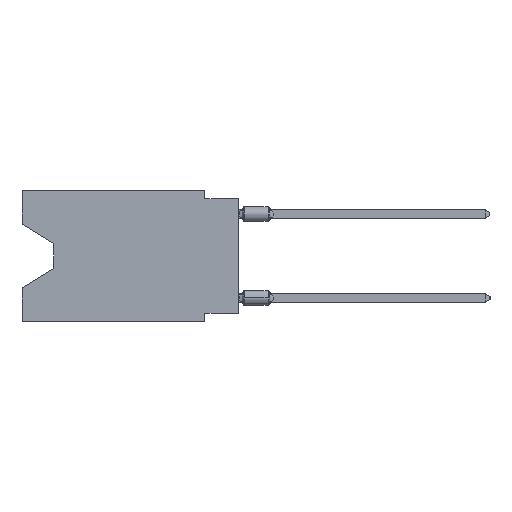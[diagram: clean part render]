
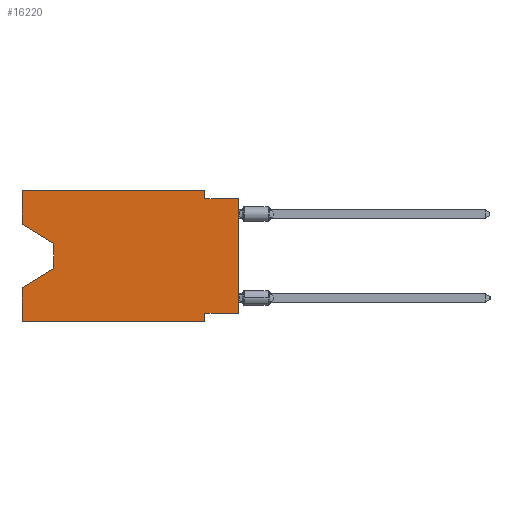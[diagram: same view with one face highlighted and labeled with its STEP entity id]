
A CAD part, left-side view. The second image highlights one B-rep face of the part: STEP entity #16220.
In plain terms, the highlighted planar face has unit normal (-1, 0, 0).
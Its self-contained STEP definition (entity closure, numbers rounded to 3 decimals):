
#616 = CARTESIAN_POINT ( 'NONE',  ( 0., 13.97, -5.893 ) ) ;
#983 = CARTESIAN_POINT ( 'NONE',  ( 0., 2.54, -9.271 ) ) ;
#1075 = DIRECTION ( 'NONE',  ( 0., 0., -1. ) ) ;
#2833 = VECTOR ( 'NONE', #36959, 1000. ) ;
#3421 = CARTESIAN_POINT ( 'NONE',  ( 0., 2.54, -9.906 ) ) ;
#3900 = VECTOR ( 'NONE', #32434, 1000. ) ;
#3931 = CARTESIAN_POINT ( 'NONE',  ( 0., 16.383, -7.36 ) ) ;
#5086 = LINE ( 'NONE', #15065, #23702 ) ;
#5093 = EDGE_CURVE ( 'NONE', #42682, #53385, #5086, .T. ) ;
#7472 = EDGE_CURVE ( 'NONE', #53385, #42718, #52020, .T. ) ;
#8225 = DIRECTION ( 'NONE',  ( 0., 1., 0. ) ) ;
#8436 = VECTOR ( 'NONE', #25805, 1000. ) ;
#8638 = VERTEX_POINT ( 'NONE', #43195 ) ;
#10455 = CARTESIAN_POINT ( 'NONE',  ( 0., 16.383, -2.546 ) ) ;
#12105 = ORIENTED_EDGE ( 'NONE', *, *, #20989, .F. ) ;
#12547 = AXIS2_PLACEMENT_3D ( 'NONE', #41620, #37340, #46183 ) ;
#12833 = VERTEX_POINT ( 'NONE', #31574 ) ;
#13502 = ORIENTED_EDGE ( 'NONE', *, *, #22454, .F. ) ;
#13740 = VERTEX_POINT ( 'NONE', #29883 ) ;
#15065 = CARTESIAN_POINT ( 'NONE',  ( 0., 13.97, -4.013 ) ) ;
#15202 = VECTOR ( 'NONE', #32832, 1000. ) ;
#15696 = EDGE_CURVE ( 'NONE', #24211, #42315, #35814, .T. ) ;
#16220 = ADVANCED_FACE ( 'NONE', ( #50727 ), #45907, .F. ) ;
#16223 = CARTESIAN_POINT ( 'NONE',  ( 0., 13.97, -4.013 ) ) ;
#16943 = LINE ( 'NONE', #34350, #38296 ) ;
#17104 = VECTOR ( 'NONE', #22099, 1000. ) ;
#18190 = EDGE_CURVE ( 'NONE', #28792, #37024, #47528, .T. ) ;
#19457 = ORIENTED_EDGE ( 'NONE', *, *, #7472, .T. ) ;
#20500 = LINE ( 'NONE', #24783, #28545 ) ;
#20989 = EDGE_CURVE ( 'NONE', #24211, #42718, #32945, .T. ) ;
#21168 = VECTOR ( 'NONE', #54066, 1000. ) ;
#21822 = DIRECTION ( 'NONE',  ( 0., -1., 0. ) ) ;
#21940 = VECTOR ( 'NONE', #52589, 1000. ) ;
#22099 = DIRECTION ( 'NONE',  ( 0., -1., 0. ) ) ;
#22454 = EDGE_CURVE ( 'NONE', #26311, #42315, #46953, .T. ) ;
#23299 = CARTESIAN_POINT ( 'NONE',  ( 0., 0., 0. ) ) ;
#23369 = VERTEX_POINT ( 'NONE', #10455 ) ;
#23702 = VECTOR ( 'NONE', #1075, 1000. ) ;
#23975 = LINE ( 'NONE', #45688, #15202 ) ;
#24032 = ORIENTED_EDGE ( 'NONE', *, *, #15696, .T. ) ;
#24211 = VERTEX_POINT ( 'NONE', #40010 ) ;
#24511 = VECTOR ( 'NONE', #21822, 1000. ) ;
#24609 = EDGE_CURVE ( 'NONE', #12833, #37024, #54378, .T. ) ;
#24650 = LINE ( 'NONE', #46356, #21168 ) ;
#24783 = CARTESIAN_POINT ( 'NONE',  ( 0., 0., -9.271 ) ) ;
#25805 = DIRECTION ( 'NONE',  ( 0., 0., -1. ) ) ;
#26311 = VERTEX_POINT ( 'NONE', #983 ) ;
#26317 = CARTESIAN_POINT ( 'NONE',  ( 0., 13.97, -5.893 ) ) ;
#27754 = ORIENTED_EDGE ( 'NONE', *, *, #46187, .F. ) ;
#28314 = ORIENTED_EDGE ( 'NONE', *, *, #5093, .T. ) ;
#28426 = ORIENTED_EDGE ( 'NONE', *, *, #24609, .T. ) ;
#28545 = VECTOR ( 'NONE', #8225, 1000. ) ;
#28792 = VERTEX_POINT ( 'NONE', #43923 ) ;
#29199 = LINE ( 'NONE', #39190, #33894 ) ;
#29632 = EDGE_CURVE ( 'NONE', #23369, #42682, #23975, .T. ) ;
#29848 = ORIENTED_EDGE ( 'NONE', *, *, #36684, .F. ) ;
#29883 = CARTESIAN_POINT ( 'NONE',  ( 0., 2.54, 0. ) ) ;
#31574 = CARTESIAN_POINT ( 'NONE',  ( 0., 0., -9.271 ) ) ;
#32434 = DIRECTION ( 'NONE',  ( 0., 0., 1. ) ) ;
#32832 = DIRECTION ( 'NONE',  ( 0., -0.855, -0.519 ) ) ;
#32945 = LINE ( 'NONE', #41230, #2833 ) ;
#33894 = VECTOR ( 'NONE', #38634, 1000. ) ;
#34096 = CARTESIAN_POINT ( 'NONE',  ( 0., 2.54, -9.906 ) ) ;
#34350 = CARTESIAN_POINT ( 'NONE',  ( 0., 2.54, 0. ) ) ;
#35722 = ORIENTED_EDGE ( 'NONE', *, *, #39724, .F. ) ;
#35814 = LINE ( 'NONE', #47522, #17104 ) ;
#36684 = EDGE_CURVE ( 'NONE', #8638, #13740, #29199, .T. ) ;
#36959 = DIRECTION ( 'NONE',  ( 0., 0., 1. ) ) ;
#37024 = VERTEX_POINT ( 'NONE', #42551 ) ;
#37340 = DIRECTION ( 'NONE',  ( 1., 0., 0. ) ) ;
#38296 = VECTOR ( 'NONE', #42909, 1000. ) ;
#38634 = DIRECTION ( 'NONE',  ( 0., -1., 0. ) ) ;
#39190 = CARTESIAN_POINT ( 'NONE',  ( 0., 16.383, 0. ) ) ;
#39724 = EDGE_CURVE ( 'NONE', #12833, #26311, #20500, .T. ) ;
#40010 = CARTESIAN_POINT ( 'NONE',  ( 0., 16.383, -9.906 ) ) ;
#41230 = CARTESIAN_POINT ( 'NONE',  ( 0., 16.383, 0. ) ) ;
#41620 = CARTESIAN_POINT ( 'NONE',  ( 0., 16.383, 0. ) ) ;
#42315 = VERTEX_POINT ( 'NONE', #3421 ) ;
#42551 = CARTESIAN_POINT ( 'NONE',  ( 0., 0., -0.635 ) ) ;
#42682 = VERTEX_POINT ( 'NONE', #16223 ) ;
#42718 = VERTEX_POINT ( 'NONE', #3931 ) ;
#42909 = DIRECTION ( 'NONE',  ( 0., 0., -1. ) ) ;
#43195 = CARTESIAN_POINT ( 'NONE',  ( 0., 16.383, 0. ) ) ;
#43218 = EDGE_CURVE ( 'NONE', #13740, #28792, #16943, .T. ) ;
#43923 = CARTESIAN_POINT ( 'NONE',  ( 0., 2.54, -0.635 ) ) ;
#44887 = ORIENTED_EDGE ( 'NONE', *, *, #43218, .F. ) ;
#45688 = CARTESIAN_POINT ( 'NONE',  ( 0., 16.383, -2.546 ) ) ;
#45907 = PLANE ( 'NONE',  #12547 ) ;
#46183 = DIRECTION ( 'NONE',  ( 0., 0., -1. ) ) ;
#46187 = EDGE_CURVE ( 'NONE', #23369, #8638, #24650, .T. ) ;
#46356 = CARTESIAN_POINT ( 'NONE',  ( 0., 16.383, 0. ) ) ;
#46953 = LINE ( 'NONE', #34096, #8436 ) ;
#47385 = ORIENTED_EDGE ( 'NONE', *, *, #29632, .T. ) ;
#47522 = CARTESIAN_POINT ( 'NONE',  ( 0., 16.383, -9.906 ) ) ;
#47528 = LINE ( 'NONE', #51790, #24511 ) ;
#48037 = EDGE_LOOP ( 'NONE', ( #47385, #28314, #19457, #12105, #24032, #13502, #35722, #28426, #51346, #44887, #29848, #27754 ) ) ;
#50727 = FACE_OUTER_BOUND ( 'NONE', #48037, .T. ) ;
#51346 = ORIENTED_EDGE ( 'NONE', *, *, #18190, .F. ) ;
#51790 = CARTESIAN_POINT ( 'NONE',  ( 0., 0., -0.635 ) ) ;
#52020 = LINE ( 'NONE', #616, #21940 ) ;
#52589 = DIRECTION ( 'NONE',  ( 0., 0.855, -0.519 ) ) ;
#53385 = VERTEX_POINT ( 'NONE', #26317 ) ;
#54066 = DIRECTION ( 'NONE',  ( 0., 0., 1. ) ) ;
#54378 = LINE ( 'NONE', #23299, #3900 ) ;
